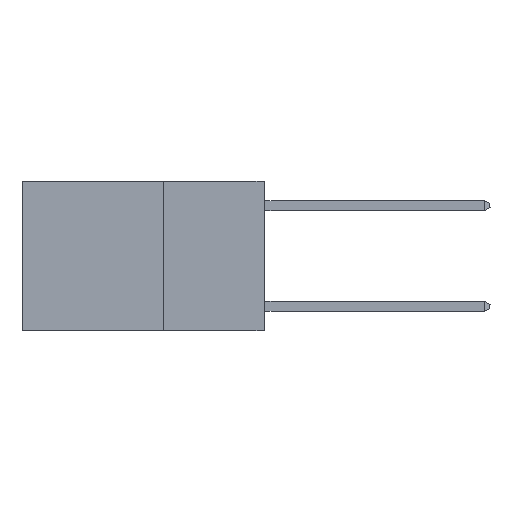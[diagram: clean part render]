
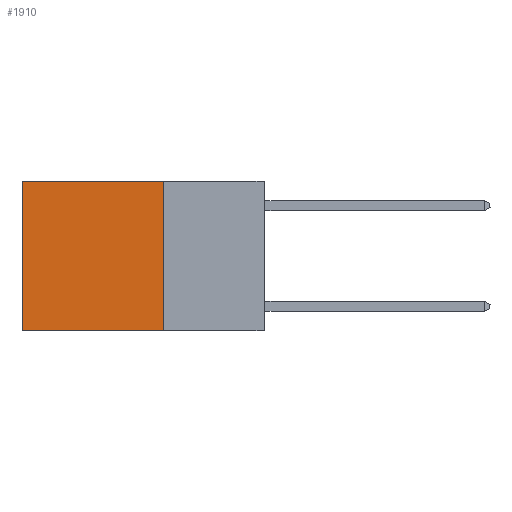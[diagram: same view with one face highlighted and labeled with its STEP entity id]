
A CAD part, left-side view. The second image highlights one B-rep face of the part: STEP entity #1910.
In plain terms, the highlighted planar face has unit normal (-1, 0, 0).
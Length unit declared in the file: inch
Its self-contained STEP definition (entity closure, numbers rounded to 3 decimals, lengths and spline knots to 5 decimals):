
#720 = VECTOR ( 'NONE', #19790, 39.37008 ) ;
#1425 = LINE ( 'NONE', #12486, #1513 ) ;
#1513 = VECTOR ( 'NONE', #19352, 39.37008 ) ;
#1877 = CARTESIAN_POINT ( 'NONE',  ( 0.2625, 0.25, 0. ) ) ;
#1910 = ADVANCED_FACE ( 'NONE', ( #25722 ), #5599, .F. ) ;
#2115 = CARTESIAN_POINT ( 'NONE',  ( 0.2625, 0.25, 0. ) ) ;
#2659 = ORIENTED_EDGE ( 'NONE', *, *, #20985, .F. ) ;
#4084 = AXIS2_PLACEMENT_3D ( 'NONE', #25117, #23496, #27313 ) ;
#4306 = LINE ( 'NONE', #2115, #19015 ) ;
#5599 = PLANE ( 'NONE',  #4084 ) ;
#5808 = LINE ( 'NONE', #26077, #20890 ) ;
#6232 = EDGE_CURVE ( 'NONE', #28882, #8828, #1425, .T. ) ;
#8530 = ORIENTED_EDGE ( 'NONE', *, *, #27326, .T. ) ;
#8828 = VERTEX_POINT ( 'NONE', #19120 ) ;
#9131 = VERTEX_POINT ( 'NONE', #22850 ) ;
#12086 = ORIENTED_EDGE ( 'NONE', *, *, #21090, .F. ) ;
#12167 = DIRECTION ( 'NONE',  ( 0., 1., 0. ) ) ;
#12486 = CARTESIAN_POINT ( 'NONE',  ( 0.2625, 0.6, 0. ) ) ;
#18702 = CARTESIAN_POINT ( 'NONE',  ( 0.2625, 0.6, 0. ) ) ;
#19015 = VECTOR ( 'NONE', #26670, 39.37008 ) ;
#19120 = CARTESIAN_POINT ( 'NONE',  ( 0.2625, 0.6, -0.37 ) ) ;
#19352 = DIRECTION ( 'NONE',  ( 0., 0., -1. ) ) ;
#19790 = DIRECTION ( 'NONE',  ( 0., 1., 0. ) ) ;
#20890 = VECTOR ( 'NONE', #12167, 39.37008 ) ;
#20985 = EDGE_CURVE ( 'NONE', #9131, #8828, #5808, .T. ) ;
#21090 = EDGE_CURVE ( 'NONE', #25155, #9131, #4306, .T. ) ;
#22015 = LINE ( 'NONE', #1877, #720 ) ;
#22850 = CARTESIAN_POINT ( 'NONE',  ( 0.2625, 0.25, -0.37 ) ) ;
#23392 = ORIENTED_EDGE ( 'NONE', *, *, #6232, .T. ) ;
#23496 = DIRECTION ( 'NONE',  ( 1., 0., 0. ) ) ;
#23575 = EDGE_LOOP ( 'NONE', ( #23392, #2659, #12086, #8530 ) ) ;
#25117 = CARTESIAN_POINT ( 'NONE',  ( 0.2625, 0.25, 0. ) ) ;
#25155 = VERTEX_POINT ( 'NONE', #27574 ) ;
#25722 = FACE_OUTER_BOUND ( 'NONE', #23575, .T. ) ;
#26077 = CARTESIAN_POINT ( 'NONE',  ( 0.2625, 0.25, -0.37 ) ) ;
#26670 = DIRECTION ( 'NONE',  ( 0., 0., -1. ) ) ;
#27313 = DIRECTION ( 'NONE',  ( 0., 0., -1. ) ) ;
#27326 = EDGE_CURVE ( 'NONE', #25155, #28882, #22015, .T. ) ;
#27574 = CARTESIAN_POINT ( 'NONE',  ( 0.2625, 0.25, 0. ) ) ;
#28882 = VERTEX_POINT ( 'NONE', #18702 ) ;
